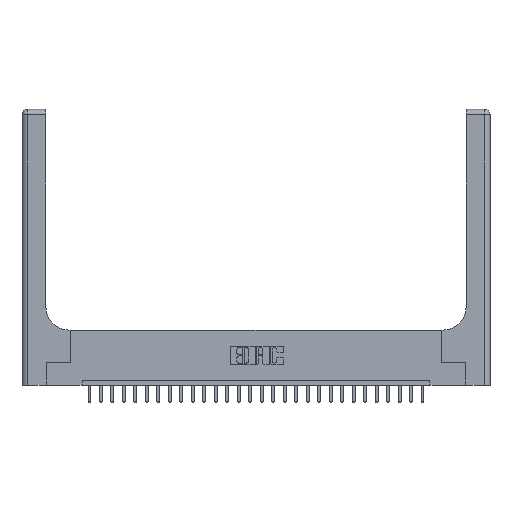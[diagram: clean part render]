
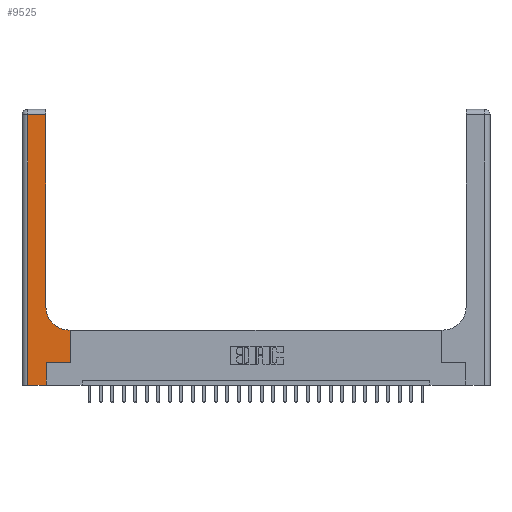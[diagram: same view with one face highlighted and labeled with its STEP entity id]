
A CAD part, top view. The second image highlights one B-rep face of the part: STEP entity #9525.
In plain terms, the highlighted planar face has unit normal (0, 0, 1).
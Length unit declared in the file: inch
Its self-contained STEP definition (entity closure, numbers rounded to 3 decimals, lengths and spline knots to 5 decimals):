
#220 = CARTESIAN_POINT ( 'NONE',  ( 0.528, 0.25, 0.37 ) ) ;
#886 = CARTESIAN_POINT ( 'NONE',  ( 0., 0., 0.37 ) ) ;
#1037 = VECTOR ( 'NONE', #23803, 39.37008 ) ;
#1490 = CARTESIAN_POINT ( 'NONE',  ( 0., 2.94, 0.37 ) ) ;
#1811 = DIRECTION ( 'NONE',  ( 0., -1., 0. ) ) ;
#2107 = CARTESIAN_POINT ( 'NONE',  ( 0.265, 0., 0.37 ) ) ;
#2524 = EDGE_LOOP ( 'NONE', ( #18973, #16808, #23428, #5966, #7053, #11686, #11717, #18697, #17775 ) ) ;
#2736 = LINE ( 'NONE', #21536, #16935 ) ;
#3035 = CARTESIAN_POINT ( 'NONE',  ( 0.265, 0.25, 0.37 ) ) ;
#3417 = CARTESIAN_POINT ( 'NONE',  ( 0.26, 2.94, 0.37 ) ) ;
#3941 = EDGE_CURVE ( 'NONE', #23811, #16892, #22009, .T. ) ;
#3983 = CARTESIAN_POINT ( 'NONE',  ( 0.265, 0.25, 0.37 ) ) ;
#4056 = LINE ( 'NONE', #21413, #12449 ) ;
#5266 = EDGE_CURVE ( 'NONE', #18450, #11761, #16525, .T. ) ;
#5283 = AXIS2_PLACEMENT_3D ( 'NONE', #11565, #17391, #25375 ) ;
#5966 = ORIENTED_EDGE ( 'NONE', *, *, #18570, .T. ) ;
#6287 = AXIS2_PLACEMENT_3D ( 'NONE', #7597, #23308, #13648 ) ;
#6361 = VERTEX_POINT ( 'NONE', #3983 ) ;
#6658 = LINE ( 'NONE', #11819, #1037 ) ;
#7053 = ORIENTED_EDGE ( 'NONE', *, *, #10301, .T. ) ;
#7331 = DIRECTION ( 'NONE',  ( -1., 0., 0. ) ) ;
#7597 = CARTESIAN_POINT ( 'NONE',  ( 0.51, 0.85, 0.37 ) ) ;
#7794 = DIRECTION ( 'NONE',  ( 0., 1., 0. ) ) ;
#7884 = DIRECTION ( 'NONE',  ( 0., 1., 0. ) ) ;
#7975 = EDGE_CURVE ( 'NONE', #11761, #23384, #12048, .T. ) ;
#8646 = EDGE_CURVE ( 'NONE', #16892, #16467, #2736, .T. ) ;
#8839 = VECTOR ( 'NONE', #7331, 39.37008 ) ;
#9005 = DIRECTION ( 'NONE',  ( -1., 0., 0. ) ) ;
#9037 = DIRECTION ( 'NONE',  ( 1., 0., 0. ) ) ;
#9525 = ADVANCED_FACE ( 'NONE', ( #15351 ), #21381, .F. ) ;
#9732 = CARTESIAN_POINT ( 'NONE',  ( 0.26, 0.85, 0.37 ) ) ;
#10301 = EDGE_CURVE ( 'NONE', #20292, #6361, #22979, .T. ) ;
#10343 = CARTESIAN_POINT ( 'NONE',  ( 0.26, 0.6, 0.37 ) ) ;
#10704 = EDGE_CURVE ( 'NONE', #6361, #21219, #14168, .T. ) ;
#10883 = DIRECTION ( 'NONE',  ( 1., 0., 0. ) ) ;
#11236 = CARTESIAN_POINT ( 'NONE',  ( 0.265, 0., 0.37 ) ) ;
#11315 = VECTOR ( 'NONE', #9005, 39.37008 ) ;
#11565 = CARTESIAN_POINT ( 'NONE',  ( 0., 3., 0.37 ) ) ;
#11686 = ORIENTED_EDGE ( 'NONE', *, *, #10704, .T. ) ;
#11717 = ORIENTED_EDGE ( 'NONE', *, *, #22351, .T. ) ;
#11761 = VERTEX_POINT ( 'NONE', #16377 ) ;
#11819 = CARTESIAN_POINT ( 'NONE',  ( 0.528, 0.25, 0.37 ) ) ;
#12048 = CIRCLE ( 'NONE', #6287, 0.25 ) ;
#12199 = CARTESIAN_POINT ( 'NONE',  ( 0.06, 0., 0.37 ) ) ;
#12449 = VECTOR ( 'NONE', #7794, 39.37008 ) ;
#13648 = DIRECTION ( 'NONE',  ( 1., 0., 0. ) ) ;
#13944 = VECTOR ( 'NONE', #10883, 39.37008 ) ;
#14168 = LINE ( 'NONE', #3035, #15145 ) ;
#14536 = LINE ( 'NONE', #886, #13944 ) ;
#15145 = VECTOR ( 'NONE', #9037, 39.37008 ) ;
#15351 = FACE_OUTER_BOUND ( 'NONE', #2524, .T. ) ;
#16377 = CARTESIAN_POINT ( 'NONE',  ( 0.51, 0.6, 0.37 ) ) ;
#16467 = VERTEX_POINT ( 'NONE', #12199 ) ;
#16474 = CARTESIAN_POINT ( 'NONE',  ( 0.06, 2.94, 0.37 ) ) ;
#16525 = LINE ( 'NONE', #10343, #11315 ) ;
#16808 = ORIENTED_EDGE ( 'NONE', *, *, #3941, .T. ) ;
#16892 = VERTEX_POINT ( 'NONE', #16474 ) ;
#16935 = VECTOR ( 'NONE', #1811, 39.37008 ) ;
#17391 = DIRECTION ( 'NONE',  ( 0., 0., -1. ) ) ;
#17775 = ORIENTED_EDGE ( 'NONE', *, *, #7975, .T. ) ;
#18450 = VERTEX_POINT ( 'NONE', #22258 ) ;
#18570 = EDGE_CURVE ( 'NONE', #16467, #20292, #14536, .T. ) ;
#18697 = ORIENTED_EDGE ( 'NONE', *, *, #5266, .T. ) ;
#18973 = ORIENTED_EDGE ( 'NONE', *, *, #23882, .T. ) ;
#20292 = VERTEX_POINT ( 'NONE', #11236 ) ;
#21112 = VECTOR ( 'NONE', #7884, 39.37008 ) ;
#21219 = VERTEX_POINT ( 'NONE', #220 ) ;
#21381 = PLANE ( 'NONE',  #5283 ) ;
#21413 = CARTESIAN_POINT ( 'NONE',  ( 0.26, 3., 0.37 ) ) ;
#21536 = CARTESIAN_POINT ( 'NONE',  ( 0.06, 3., 0.37 ) ) ;
#22009 = LINE ( 'NONE', #1490, #8839 ) ;
#22258 = CARTESIAN_POINT ( 'NONE',  ( 0.528, 0.6, 0.37 ) ) ;
#22351 = EDGE_CURVE ( 'NONE', #21219, #18450, #6658, .T. ) ;
#22979 = LINE ( 'NONE', #2107, #21112 ) ;
#23308 = DIRECTION ( 'NONE',  ( 0., 0., -1. ) ) ;
#23384 = VERTEX_POINT ( 'NONE', #9732 ) ;
#23428 = ORIENTED_EDGE ( 'NONE', *, *, #8646, .T. ) ;
#23803 = DIRECTION ( 'NONE',  ( 0., 1., 0. ) ) ;
#23811 = VERTEX_POINT ( 'NONE', #3417 ) ;
#23882 = EDGE_CURVE ( 'NONE', #23384, #23811, #4056, .T. ) ;
#25375 = DIRECTION ( 'NONE',  ( -1., 0., 0. ) ) ;
